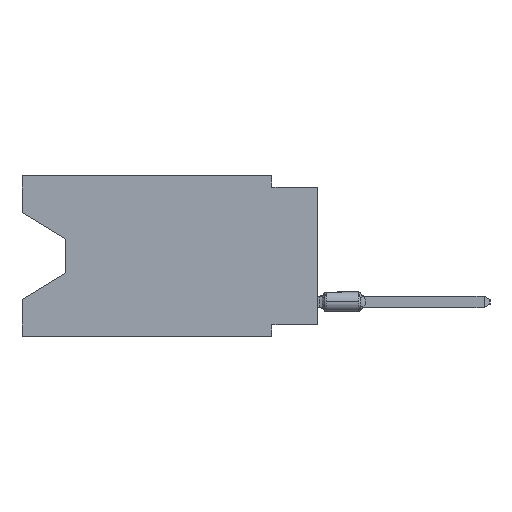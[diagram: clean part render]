
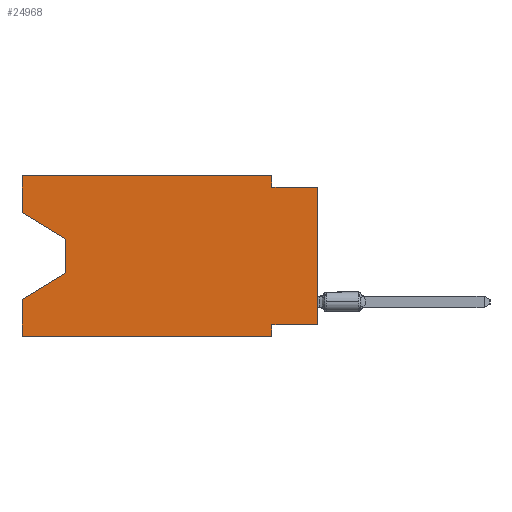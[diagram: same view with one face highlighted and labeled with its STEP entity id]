
A CAD part, left-side view. The second image highlights one B-rep face of the part: STEP entity #24968.
In plain terms, the highlighted planar face has unit normal (-1, 0, 0).
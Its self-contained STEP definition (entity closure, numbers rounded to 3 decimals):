
#60 = EDGE_CURVE ( 'NONE', #24134, #18126, #321, .T. ) ;
#321 = LINE ( 'NONE', #2454, #11152 ) ;
#382 = ORIENTED_EDGE ( 'NONE', *, *, #16268, .F. ) ;
#1272 = EDGE_CURVE ( 'NONE', #9108, #15781, #22155, .T. ) ;
#1387 = VECTOR ( 'NONE', #16997, 1000. ) ;
#1559 = CARTESIAN_POINT ( 'NONE',  ( 0., 16.383, -8.89 ) ) ;
#1979 = DIRECTION ( 'NONE',  ( 0., -0.855, -0.519 ) ) ;
#2180 = CARTESIAN_POINT ( 'NONE',  ( 0., 2.54, 0. ) ) ;
#2340 = VECTOR ( 'NONE', #31296, 1000. ) ;
#2454 = CARTESIAN_POINT ( 'NONE',  ( 0., 0., -0.635 ) ) ;
#3161 = VERTEX_POINT ( 'NONE', #16071 ) ;
#3608 = LINE ( 'NONE', #6031, #11356 ) ;
#5422 = VECTOR ( 'NONE', #1979, 1000. ) ;
#6031 = CARTESIAN_POINT ( 'NONE',  ( 0., 0., 0. ) ) ;
#6101 = CARTESIAN_POINT ( 'NONE',  ( 0., 0., -0.635 ) ) ;
#6201 = EDGE_CURVE ( 'NONE', #30534, #15781, #20053, .T. ) ;
#7354 = DIRECTION ( 'NONE',  ( 0., 0., -1. ) ) ;
#7464 = LINE ( 'NONE', #22883, #25696 ) ;
#7913 = DIRECTION ( 'NONE',  ( 0., -1., 0. ) ) ;
#7933 = VERTEX_POINT ( 'NONE', #2180 ) ;
#8008 = DIRECTION ( 'NONE',  ( 0., 0., -1. ) ) ;
#8827 = FACE_OUTER_BOUND ( 'NONE', #20604, .T. ) ;
#8875 = LINE ( 'NONE', #18973, #16725 ) ;
#9041 = DIRECTION ( 'NONE',  ( 0., -1., 0. ) ) ;
#9108 = VERTEX_POINT ( 'NONE', #1559 ) ;
#9553 = EDGE_CURVE ( 'NONE', #11749, #3161, #30420, .T. ) ;
#10936 = CARTESIAN_POINT ( 'NONE',  ( 0., 2.54, 0. ) ) ;
#11152 = VECTOR ( 'NONE', #7913, 1000. ) ;
#11356 = VECTOR ( 'NONE', #15933, 1000. ) ;
#11399 = EDGE_CURVE ( 'NONE', #14755, #11749, #30811, .T. ) ;
#11744 = ORIENTED_EDGE ( 'NONE', *, *, #9553, .T. ) ;
#11749 = VERTEX_POINT ( 'NONE', #19138 ) ;
#11925 = DIRECTION ( 'NONE',  ( 1., 0., 0. ) ) ;
#12000 = DIRECTION ( 'NONE',  ( 0., 0., -1. ) ) ;
#12016 = LINE ( 'NONE', #24352, #5422 ) ;
#12306 = VECTOR ( 'NONE', #12747, 1000. ) ;
#12747 = DIRECTION ( 'NONE',  ( 0., 0.855, -0.519 ) ) ;
#12819 = VERTEX_POINT ( 'NONE', #30798 ) ;
#13173 = CARTESIAN_POINT ( 'NONE',  ( 0., 13.97, -3.505 ) ) ;
#13255 = ORIENTED_EDGE ( 'NONE', *, *, #14380, .F. ) ;
#13926 = CARTESIAN_POINT ( 'NONE',  ( 0., 0., -8.255 ) ) ;
#13959 = CARTESIAN_POINT ( 'NONE',  ( 0., 2.54, -0.635 ) ) ;
#14291 = LINE ( 'NONE', #17046, #2340 ) ;
#14380 = EDGE_CURVE ( 'NONE', #7933, #24134, #23427, .T. ) ;
#14755 = VERTEX_POINT ( 'NONE', #13173 ) ;
#15111 = ORIENTED_EDGE ( 'NONE', *, *, #25532, .F. ) ;
#15434 = CARTESIAN_POINT ( 'NONE',  ( 0., 2.54, -8.255 ) ) ;
#15577 = EDGE_CURVE ( 'NONE', #29616, #18126, #3608, .T. ) ;
#15705 = CARTESIAN_POINT ( 'NONE',  ( 0., 0., -8.255 ) ) ;
#15781 = VERTEX_POINT ( 'NONE', #28089 ) ;
#15933 = DIRECTION ( 'NONE',  ( 0., 0., 1. ) ) ;
#16071 = CARTESIAN_POINT ( 'NONE',  ( 0., 16.383, -6.852 ) ) ;
#16073 = ORIENTED_EDGE ( 'NONE', *, *, #16652, .F. ) ;
#16268 = EDGE_CURVE ( 'NONE', #9108, #3161, #14291, .T. ) ;
#16506 = VERTEX_POINT ( 'NONE', #28340 ) ;
#16652 = EDGE_CURVE ( 'NONE', #29616, #30534, #18963, .T. ) ;
#16725 = VECTOR ( 'NONE', #9041, 1000. ) ;
#16872 = AXIS2_PLACEMENT_3D ( 'NONE', #31539, #11925, #7354 ) ;
#16997 = DIRECTION ( 'NONE',  ( 0., 0., -1. ) ) ;
#17046 = CARTESIAN_POINT ( 'NONE',  ( 0., 16.383, 0. ) ) ;
#17114 = PLANE ( 'NONE',  #16872 ) ;
#17386 = DIRECTION ( 'NONE',  ( 0., 0., 1. ) ) ;
#17475 = EDGE_CURVE ( 'NONE', #16506, #14755, #12016, .T. ) ;
#18126 = VERTEX_POINT ( 'NONE', #6101 ) ;
#18174 = VECTOR ( 'NONE', #8008, 1000. ) ;
#18618 = ORIENTED_EDGE ( 'NONE', *, *, #15577, .T. ) ;
#18963 = LINE ( 'NONE', #13926, #19387 ) ;
#18973 = CARTESIAN_POINT ( 'NONE',  ( 0., 16.383, 0. ) ) ;
#19138 = CARTESIAN_POINT ( 'NONE',  ( 0., 13.97, -5.385 ) ) ;
#19387 = VECTOR ( 'NONE', #24156, 1000. ) ;
#20053 = LINE ( 'NONE', #29933, #1387 ) ;
#20284 = ORIENTED_EDGE ( 'NONE', *, *, #21580, .F. ) ;
#20604 = EDGE_LOOP ( 'NONE', ( #22624, #28238, #11744, #382, #21204, #26058, #16073, #18618, #22310, #13255, #20284, #15111 ) ) ;
#21204 = ORIENTED_EDGE ( 'NONE', *, *, #1272, .T. ) ;
#21479 = VECTOR ( 'NONE', #24280, 1000. ) ;
#21580 = EDGE_CURVE ( 'NONE', #12819, #7933, #8875, .T. ) ;
#21833 = CARTESIAN_POINT ( 'NONE',  ( 0., 16.383, -8.89 ) ) ;
#22155 = LINE ( 'NONE', #21833, #21479 ) ;
#22310 = ORIENTED_EDGE ( 'NONE', *, *, #60, .F. ) ;
#22624 = ORIENTED_EDGE ( 'NONE', *, *, #17475, .T. ) ;
#22883 = CARTESIAN_POINT ( 'NONE',  ( 0., 16.383, 0. ) ) ;
#23427 = LINE ( 'NONE', #10936, #18174 ) ;
#24134 = VERTEX_POINT ( 'NONE', #13959 ) ;
#24156 = DIRECTION ( 'NONE',  ( 0., 1., 0. ) ) ;
#24280 = DIRECTION ( 'NONE',  ( 0., -1., 0. ) ) ;
#24352 = CARTESIAN_POINT ( 'NONE',  ( 0., 16.383, -2.038 ) ) ;
#24800 = VECTOR ( 'NONE', #12000, 1000. ) ;
#24968 = ADVANCED_FACE ( 'NONE', ( #8827 ), #17114, .F. ) ;
#25532 = EDGE_CURVE ( 'NONE', #16506, #12819, #7464, .T. ) ;
#25696 = VECTOR ( 'NONE', #17386, 1000. ) ;
#26058 = ORIENTED_EDGE ( 'NONE', *, *, #6201, .F. ) ;
#27366 = CARTESIAN_POINT ( 'NONE',  ( 0., 13.97, -3.505 ) ) ;
#28089 = CARTESIAN_POINT ( 'NONE',  ( 0., 2.54, -8.89 ) ) ;
#28238 = ORIENTED_EDGE ( 'NONE', *, *, #11399, .T. ) ;
#28284 = CARTESIAN_POINT ( 'NONE',  ( 0., 13.97, -5.385 ) ) ;
#28340 = CARTESIAN_POINT ( 'NONE',  ( 0., 16.383, -2.038 ) ) ;
#29616 = VERTEX_POINT ( 'NONE', #15705 ) ;
#29933 = CARTESIAN_POINT ( 'NONE',  ( 0., 2.54, -8.89 ) ) ;
#30420 = LINE ( 'NONE', #28284, #12306 ) ;
#30534 = VERTEX_POINT ( 'NONE', #15434 ) ;
#30798 = CARTESIAN_POINT ( 'NONE',  ( 0., 16.383, 0. ) ) ;
#30811 = LINE ( 'NONE', #27366, #24800 ) ;
#31296 = DIRECTION ( 'NONE',  ( 0., 0., 1. ) ) ;
#31539 = CARTESIAN_POINT ( 'NONE',  ( 0., 16.383, 0. ) ) ;
